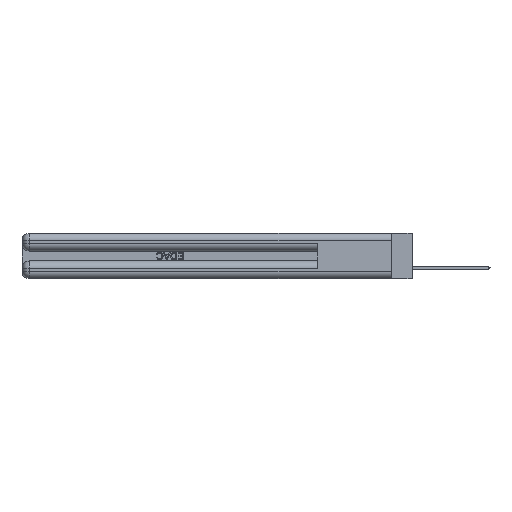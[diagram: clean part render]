
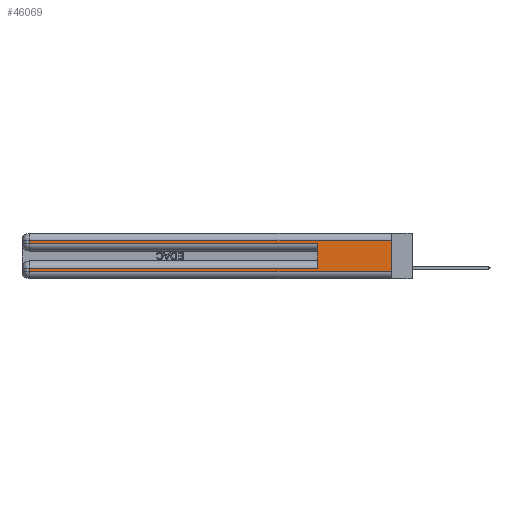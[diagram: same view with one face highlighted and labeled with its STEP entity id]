
A CAD part, left-side view. The second image highlights one B-rep face of the part: STEP entity #46069.
In plain terms, the highlighted planar face has unit normal (-1, 0, 0).
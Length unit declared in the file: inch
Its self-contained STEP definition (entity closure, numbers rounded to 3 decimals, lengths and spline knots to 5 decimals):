
#295 = VECTOR ( 'NONE', #33437, 39.37008 ) ;
#380 = DIRECTION ( 'NONE',  ( 0., 0., 1. ) ) ;
#1466 = LINE ( 'NONE', #26250, #295 ) ;
#2452 = DIRECTION ( 'NONE',  ( 0., 0., -1. ) ) ;
#2836 = ORIENTED_EDGE ( 'NONE', *, *, #22874, .T. ) ;
#3800 = LINE ( 'NONE', #38818, #19832 ) ;
#3857 = EDGE_CURVE ( 'NONE', #14169, #18509, #18004, .T. ) ;
#4521 = DIRECTION ( 'NONE',  ( 0., 0., -1. ) ) ;
#4841 = CARTESIAN_POINT ( 'NONE',  ( 0., 2.94, 0.37 ) ) ;
#5466 = CARTESIAN_POINT ( 'NONE',  ( 0., 0., 0.31 ) ) ;
#5752 = ORIENTED_EDGE ( 'NONE', *, *, #43845, .T. ) ;
#6027 = VERTEX_POINT ( 'NONE', #40521 ) ;
#6958 = ORIENTED_EDGE ( 'NONE', *, *, #22625, .F. ) ;
#8141 = LINE ( 'NONE', #18480, #43644 ) ;
#8837 = VECTOR ( 'NONE', #4521, 39.37008 ) ;
#8864 = DIRECTION ( 'NONE',  ( 0., 0., -1. ) ) ;
#9360 = CARTESIAN_POINT ( 'NONE',  ( 0., 0.6, 0.285 ) ) ;
#9563 = PLANE ( 'NONE',  #33096 ) ;
#11131 = ORIENTED_EDGE ( 'NONE', *, *, #22177, .T. ) ;
#11770 = VERTEX_POINT ( 'NONE', #20860 ) ;
#13246 = VECTOR ( 'NONE', #380, 39.37008 ) ;
#13670 = EDGE_CURVE ( 'NONE', #21308, #6027, #8141, .T. ) ;
#13702 = VERTEX_POINT ( 'NONE', #9360 ) ;
#14122 = LINE ( 'NONE', #38179, #38734 ) ;
#14169 = VERTEX_POINT ( 'NONE', #43500 ) ;
#14302 = ORIENTED_EDGE ( 'NONE', *, *, #3857, .T. ) ;
#16765 = ORIENTED_EDGE ( 'NONE', *, *, #13670, .T. ) ;
#17386 = DIRECTION ( 'NONE',  ( 0., 0., -1. ) ) ;
#17620 = EDGE_CURVE ( 'NONE', #38630, #11770, #31824, .T. ) ;
#18004 = LINE ( 'NONE', #4841, #8837 ) ;
#18452 = CARTESIAN_POINT ( 'NONE',  ( 0., 0.6, 0.145 ) ) ;
#18480 = CARTESIAN_POINT ( 'NONE',  ( 0., 0., 0.085 ) ) ;
#18509 = VERTEX_POINT ( 'NONE', #43393 ) ;
#19832 = VECTOR ( 'NONE', #42368, 39.37008 ) ;
#19960 = CARTESIAN_POINT ( 'NONE',  ( 0., 2.94, 0.06 ) ) ;
#20860 = CARTESIAN_POINT ( 'NONE',  ( 0., 0., 0.06 ) ) ;
#21308 = VERTEX_POINT ( 'NONE', #40355 ) ;
#22177 = EDGE_CURVE ( 'NONE', #38630, #14169, #14122, .T. ) ;
#22318 = EDGE_CURVE ( 'NONE', #18509, #13702, #3800, .T. ) ;
#22625 = EDGE_CURVE ( 'NONE', #21308, #13702, #41617, .T. ) ;
#22874 = EDGE_CURVE ( 'NONE', #6027, #25709, #34433, .T. ) ;
#24259 = CARTESIAN_POINT ( 'NONE',  ( 0., 0., 0.37 ) ) ;
#24961 = FACE_OUTER_BOUND ( 'NONE', #26365, .T. ) ;
#25709 = VERTEX_POINT ( 'NONE', #19960 ) ;
#26250 = CARTESIAN_POINT ( 'NONE',  ( 0., 0., 0.06 ) ) ;
#26365 = EDGE_LOOP ( 'NONE', ( #36610, #11131, #14302, #34943, #6958, #16765, #2836, #5752 ) ) ;
#30515 = DIRECTION ( 'NONE',  ( 0., 1., 0. ) ) ;
#31824 = LINE ( 'NONE', #35246, #39879 ) ;
#33096 = AXIS2_PLACEMENT_3D ( 'NONE', #24259, #46213, #17386 ) ;
#33437 = DIRECTION ( 'NONE',  ( 0., -1., 0. ) ) ;
#34433 = LINE ( 'NONE', #34759, #47071 ) ;
#34759 = CARTESIAN_POINT ( 'NONE',  ( 0., 2.94, 0.37 ) ) ;
#34943 = ORIENTED_EDGE ( 'NONE', *, *, #22318, .T. ) ;
#35246 = CARTESIAN_POINT ( 'NONE',  ( 0., 0., 0.37 ) ) ;
#36610 = ORIENTED_EDGE ( 'NONE', *, *, #17620, .F. ) ;
#38179 = CARTESIAN_POINT ( 'NONE',  ( 0., 0., 0.31 ) ) ;
#38630 = VERTEX_POINT ( 'NONE', #5466 ) ;
#38734 = VECTOR ( 'NONE', #30515, 39.37008 ) ;
#38818 = CARTESIAN_POINT ( 'NONE',  ( 0., 0., 0.285 ) ) ;
#39879 = VECTOR ( 'NONE', #2452, 39.37008 ) ;
#40355 = CARTESIAN_POINT ( 'NONE',  ( 0., 0.6, 0.085 ) ) ;
#40521 = CARTESIAN_POINT ( 'NONE',  ( 0., 2.94, 0.085 ) ) ;
#41617 = LINE ( 'NONE', #18452, #13246 ) ;
#42368 = DIRECTION ( 'NONE',  ( 0., -1., 0. ) ) ;
#43393 = CARTESIAN_POINT ( 'NONE',  ( 0., 2.94, 0.285 ) ) ;
#43500 = CARTESIAN_POINT ( 'NONE',  ( 0., 2.94, 0.31 ) ) ;
#43644 = VECTOR ( 'NONE', #44751, 39.37008 ) ;
#43845 = EDGE_CURVE ( 'NONE', #25709, #11770, #1466, .T. ) ;
#44751 = DIRECTION ( 'NONE',  ( 0., 1., 0. ) ) ;
#46069 = ADVANCED_FACE ( 'NONE', ( #24961 ), #9563, .F. ) ;
#46213 = DIRECTION ( 'NONE',  ( 1., 0., 0. ) ) ;
#47071 = VECTOR ( 'NONE', #8864, 39.37008 ) ;
